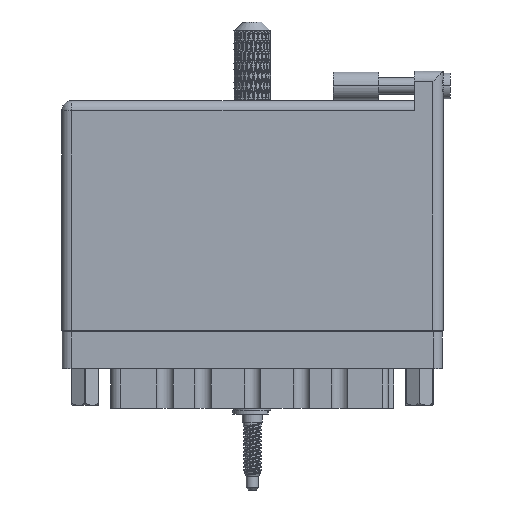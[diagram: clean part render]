
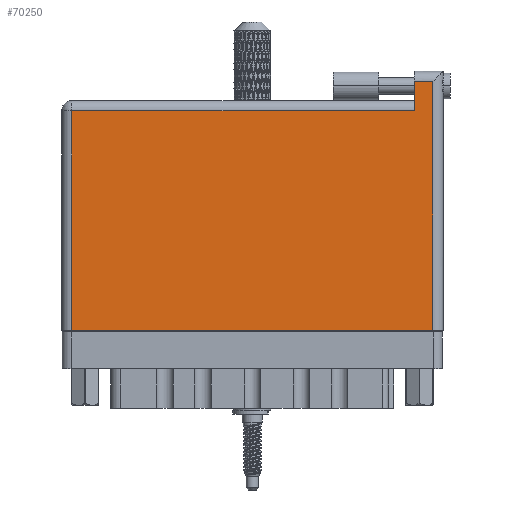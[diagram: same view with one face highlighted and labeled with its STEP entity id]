
A CAD part, front view. The second image highlights one B-rep face of the part: STEP entity #70250.
In plain terms, the highlighted face is planar.
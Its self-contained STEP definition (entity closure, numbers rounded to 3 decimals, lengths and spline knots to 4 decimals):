
#1461 = EDGE_CURVE ( 'NONE', #105392, #33555, #28045, .T. ) ;
#1859 = EDGE_CURVE ( 'NONE', #77651, #105392, #44408, .T. ) ;
#2086 = VERTEX_POINT ( 'NONE', #4561 ) ;
#4561 = CARTESIAN_POINT ( 'NONE',  ( 2.53, 0., 0. ) ) ;
#6718 = DIRECTION ( 'NONE',  ( 0., -1., 0. ) ) ;
#11308 = EDGE_CURVE ( 'NONE', #40162, #77651, #83581, .T. ) ;
#12766 = CARTESIAN_POINT ( 'NONE',  ( 0., 0., 0. ) ) ;
#15620 = EDGE_LOOP ( 'NONE', ( #20897, #87617, #68606, #81983, #42291, #35669 ) ) ;
#20897 = ORIENTED_EDGE ( 'NONE', *, *, #32256, .T. ) ;
#23420 = AXIS2_PLACEMENT_3D ( 'NONE', #54852, #102764, #45718 ) ;
#25425 = VECTOR ( 'NONE', #79878, 39.3701 ) ;
#26883 = DIRECTION ( 'NONE',  ( 0., -1., 0. ) ) ;
#28045 = LINE ( 'NONE', #94731, #56314 ) ;
#29181 = EDGE_CURVE ( 'NONE', #78859, #40162, #83220, .T. ) ;
#29308 = FACE_OUTER_BOUND ( 'NONE', #15620, .T. ) ;
#32256 = EDGE_CURVE ( 'NONE', #33555, #2086, #95043, .T. ) ;
#33555 = VERTEX_POINT ( 'NONE', #110991 ) ;
#35315 = DIRECTION ( 'NONE',  ( -1., 0., 0. ) ) ;
#35669 = ORIENTED_EDGE ( 'NONE', *, *, #1461, .T. ) ;
#35918 = CARTESIAN_POINT ( 'NONE',  ( 0.07, 1.496, 0. ) ) ;
#38131 = CARTESIAN_POINT ( 'NONE',  ( 2.403, 1.696, 0. ) ) ;
#39653 = CARTESIAN_POINT ( 'NONE',  ( 2.403, 1.496, 0. ) ) ;
#40162 = VERTEX_POINT ( 'NONE', #38131 ) ;
#42291 = ORIENTED_EDGE ( 'NONE', *, *, #1859, .T. ) ;
#42347 = CARTESIAN_POINT ( 'NONE',  ( 2.53, 1.766, 0. ) ) ;
#44408 = LINE ( 'NONE', #52140, #87646 ) ;
#45718 = DIRECTION ( 'NONE',  ( -1., 0., 0. ) ) ;
#52140 = CARTESIAN_POINT ( 'NONE',  ( 0., 1.496, 0. ) ) ;
#54852 = CARTESIAN_POINT ( 'NONE',  ( 0., 1.566, 0. ) ) ;
#56314 = VECTOR ( 'NONE', #26883, 39.3701 ) ;
#61112 = LINE ( 'NONE', #42347, #25425 ) ;
#66677 = VECTOR ( 'NONE', #117652, 39.3701 ) ;
#68606 = ORIENTED_EDGE ( 'NONE', *, *, #29181, .T. ) ;
#70250 = ADVANCED_FACE ( 'NONE', ( #29308 ), #73707, .F. ) ;
#73707 = PLANE ( 'NONE',  #23420 ) ;
#75180 = EDGE_CURVE ( 'NONE', #2086, #78859, #61112, .T. ) ;
#75783 = VECTOR ( 'NONE', #35315, 39.3701 ) ;
#77651 = VERTEX_POINT ( 'NONE', #39653 ) ;
#78859 = VERTEX_POINT ( 'NONE', #117936 ) ;
#79878 = DIRECTION ( 'NONE',  ( 0., 1., 0. ) ) ;
#81983 = ORIENTED_EDGE ( 'NONE', *, *, #11308, .T. ) ;
#82017 = CARTESIAN_POINT ( 'NONE',  ( 0., 1.696, 0. ) ) ;
#83220 = LINE ( 'NONE', #82017, #75783 ) ;
#83581 = LINE ( 'NONE', #101626, #93968 ) ;
#87617 = ORIENTED_EDGE ( 'NONE', *, *, #75180, .T. ) ;
#87646 = VECTOR ( 'NONE', #108760, 39.3701 ) ;
#93968 = VECTOR ( 'NONE', #6718, 39.3701 ) ;
#94731 = CARTESIAN_POINT ( 'NONE',  ( 0.07, 0., 0. ) ) ;
#95043 = LINE ( 'NONE', #12766, #66677 ) ;
#101626 = CARTESIAN_POINT ( 'NONE',  ( 2.403, 1.766, 0. ) ) ;
#102764 = DIRECTION ( 'NONE',  ( 0., 0., -1. ) ) ;
#105392 = VERTEX_POINT ( 'NONE', #35918 ) ;
#108760 = DIRECTION ( 'NONE',  ( -1., 0., 0. ) ) ;
#110991 = CARTESIAN_POINT ( 'NONE',  ( 0.07, 0., 0. ) ) ;
#117652 = DIRECTION ( 'NONE',  ( 1., 0., 0. ) ) ;
#117936 = CARTESIAN_POINT ( 'NONE',  ( 2.53, 1.696, 0. ) ) ;
